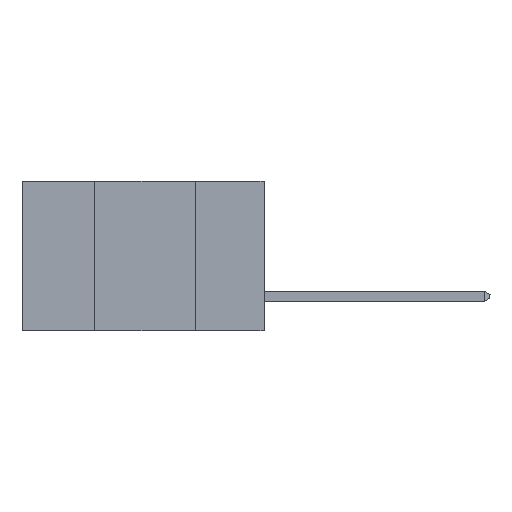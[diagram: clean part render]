
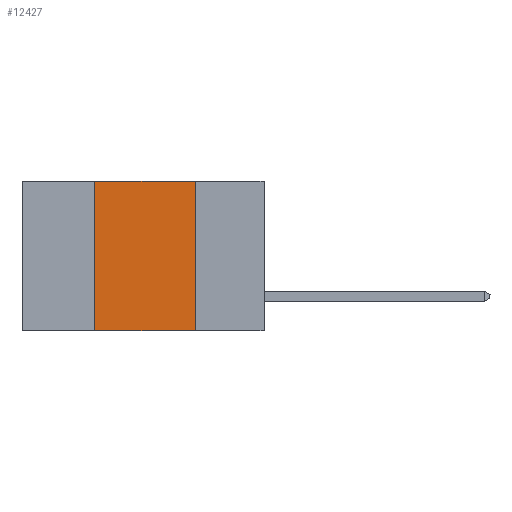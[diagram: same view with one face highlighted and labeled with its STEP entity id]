
A CAD part, left-side view. The second image highlights one B-rep face of the part: STEP entity #12427.
In plain terms, the highlighted planar face has unit normal (-1, 0, 0).
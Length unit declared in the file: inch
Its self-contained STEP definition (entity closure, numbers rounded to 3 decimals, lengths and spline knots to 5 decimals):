
#1 = EDGE_CURVE ( 'NONE', #8134, #14605, #17039, .T. ) ;
#1120 = CARTESIAN_POINT ( 'NONE',  ( 0., 0.6, 0. ) ) ;
#1290 = CARTESIAN_POINT ( 'NONE',  ( 0., 0.6, 0. ) ) ;
#1340 = CARTESIAN_POINT ( 'NONE',  ( 0., 0.17, -0.37 ) ) ;
#2713 = VECTOR ( 'NONE', #6414, 39.37008 ) ;
#2745 = DIRECTION ( 'NONE',  ( 0., 0., -1. ) ) ;
#2839 = LINE ( 'NONE', #10073, #10572 ) ;
#2992 = DIRECTION ( 'NONE',  ( 0., 0., 1. ) ) ;
#3430 = DIRECTION ( 'NONE',  ( 0., 0., -1. ) ) ;
#4198 = ORIENTED_EDGE ( 'NONE', *, *, #10859, .F. ) ;
#5280 = ORIENTED_EDGE ( 'NONE', *, *, #8924, .F. ) ;
#6256 = LINE ( 'NONE', #1120, #2713 ) ;
#6344 = CARTESIAN_POINT ( 'NONE',  ( 0., 0.17, 0. ) ) ;
#6414 = DIRECTION ( 'NONE',  ( 0., -1., 0. ) ) ;
#7572 = ORIENTED_EDGE ( 'NONE', *, *, #16420, .F. ) ;
#8078 = VECTOR ( 'NONE', #15854, 39.37008 ) ;
#8134 = VERTEX_POINT ( 'NONE', #15763 ) ;
#8907 = LINE ( 'NONE', #10990, #9936 ) ;
#8924 = EDGE_CURVE ( 'NONE', #11519, #9388, #6256, .T. ) ;
#9178 = PLANE ( 'NONE',  #11771 ) ;
#9388 = VERTEX_POINT ( 'NONE', #6344 ) ;
#9936 = VECTOR ( 'NONE', #2992, 39.37008 ) ;
#10073 = CARTESIAN_POINT ( 'NONE',  ( 0., 0.17, 0. ) ) ;
#10446 = CARTESIAN_POINT ( 'NONE',  ( 0., 0.6, -0.37 ) ) ;
#10572 = VECTOR ( 'NONE', #3430, 39.37008 ) ;
#10859 = EDGE_CURVE ( 'NONE', #8134, #11519, #8907, .T. ) ;
#10990 = CARTESIAN_POINT ( 'NONE',  ( 0., 0.42, 0. ) ) ;
#11519 = VERTEX_POINT ( 'NONE', #16382 ) ;
#11771 = AXIS2_PLACEMENT_3D ( 'NONE', #1290, #16099, #2745 ) ;
#12427 = ADVANCED_FACE ( 'NONE', ( #15489 ), #9178, .F. ) ;
#14605 = VERTEX_POINT ( 'NONE', #1340 ) ;
#14817 = EDGE_LOOP ( 'NONE', ( #7572, #5280, #4198, #16089 ) ) ;
#15489 = FACE_OUTER_BOUND ( 'NONE', #14817, .T. ) ;
#15763 = CARTESIAN_POINT ( 'NONE',  ( 0., 0.42, -0.37 ) ) ;
#15854 = DIRECTION ( 'NONE',  ( 0., -1., 0. ) ) ;
#16089 = ORIENTED_EDGE ( 'NONE', *, *, #1, .T. ) ;
#16099 = DIRECTION ( 'NONE',  ( 1., 0., 0. ) ) ;
#16382 = CARTESIAN_POINT ( 'NONE',  ( 0., 0.42, 0. ) ) ;
#16420 = EDGE_CURVE ( 'NONE', #9388, #14605, #2839, .T. ) ;
#17039 = LINE ( 'NONE', #10446, #8078 ) ;
